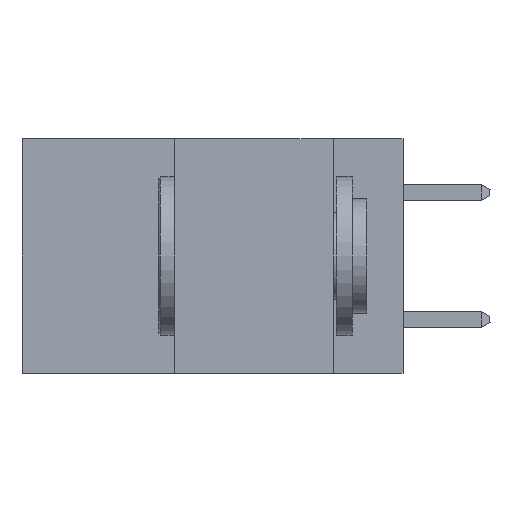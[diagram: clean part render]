
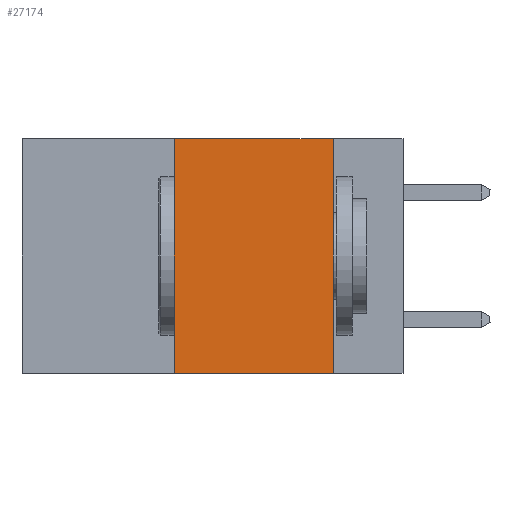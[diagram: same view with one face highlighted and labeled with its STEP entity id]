
A CAD part, left-side view. The second image highlights one B-rep face of the part: STEP entity #27174.
In plain terms, the highlighted planar face has unit normal (-1, 0, 0).
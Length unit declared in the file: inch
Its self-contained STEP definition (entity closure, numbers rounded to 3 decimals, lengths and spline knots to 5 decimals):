
#268 = DIRECTION ( 'NONE',  ( 0., 0., 1. ) ) ;
#1746 = VECTOR ( 'NONE', #5475, 39.37008 ) ;
#3232 = DIRECTION ( 'NONE',  ( 1., 0., 0. ) ) ;
#3953 = VERTEX_POINT ( 'NONE', #8296 ) ;
#4957 = ORIENTED_EDGE ( 'NONE', *, *, #16907, .F. ) ;
#5475 = DIRECTION ( 'NONE',  ( 0., -1., 0. ) ) ;
#6564 = ORIENTED_EDGE ( 'NONE', *, *, #30576, .F. ) ;
#6898 = LINE ( 'NONE', #31171, #19608 ) ;
#8201 = DIRECTION ( 'NONE',  ( 0., -1., 0. ) ) ;
#8252 = CARTESIAN_POINT ( 'NONE',  ( 0., 0.6, 0. ) ) ;
#8296 = CARTESIAN_POINT ( 'NONE',  ( 0., 0.11, -0.37 ) ) ;
#8450 = CARTESIAN_POINT ( 'NONE',  ( 0., 0.11, 0. ) ) ;
#10503 = CARTESIAN_POINT ( 'NONE',  ( 0., 0.36, 0. ) ) ;
#10897 = VERTEX_POINT ( 'NONE', #31025 ) ;
#14486 = EDGE_LOOP ( 'NONE', ( #4957, #25364, #6564, #21750 ) ) ;
#15176 = VERTEX_POINT ( 'NONE', #29341 ) ;
#15635 = LINE ( 'NONE', #8450, #28419 ) ;
#16907 = EDGE_CURVE ( 'NONE', #10897, #3953, #15635, .T. ) ;
#18574 = DIRECTION ( 'NONE',  ( 0., 0., -1. ) ) ;
#19608 = VECTOR ( 'NONE', #8201, 39.37008 ) ;
#21084 = DIRECTION ( 'NONE',  ( 0., 0., -1. ) ) ;
#21295 = EDGE_CURVE ( 'NONE', #15176, #10897, #22179, .T. ) ;
#21750 = ORIENTED_EDGE ( 'NONE', *, *, #22698, .T. ) ;
#22179 = LINE ( 'NONE', #23354, #1746 ) ;
#22698 = EDGE_CURVE ( 'NONE', #26550, #3953, #6898, .T. ) ;
#23354 = CARTESIAN_POINT ( 'NONE',  ( 0., 0.6, 0. ) ) ;
#25364 = ORIENTED_EDGE ( 'NONE', *, *, #21295, .F. ) ;
#26167 = PLANE ( 'NONE',  #30276 ) ;
#26550 = VERTEX_POINT ( 'NONE', #29048 ) ;
#27174 = ADVANCED_FACE ( 'NONE', ( #28359 ), #26167, .F. ) ;
#28359 = FACE_OUTER_BOUND ( 'NONE', #14486, .T. ) ;
#28419 = VECTOR ( 'NONE', #18574, 39.37008 ) ;
#29048 = CARTESIAN_POINT ( 'NONE',  ( 0., 0.36, -0.37 ) ) ;
#29341 = CARTESIAN_POINT ( 'NONE',  ( 0., 0.36, 0. ) ) ;
#30276 = AXIS2_PLACEMENT_3D ( 'NONE', #8252, #3232, #21084 ) ;
#30576 = EDGE_CURVE ( 'NONE', #26550, #15176, #32526, .T. ) ;
#30913 = VECTOR ( 'NONE', #268, 39.37008 ) ;
#31025 = CARTESIAN_POINT ( 'NONE',  ( 0., 0.11, 0. ) ) ;
#31171 = CARTESIAN_POINT ( 'NONE',  ( 0., 0.6, -0.37 ) ) ;
#32526 = LINE ( 'NONE', #10503, #30913 ) ;
